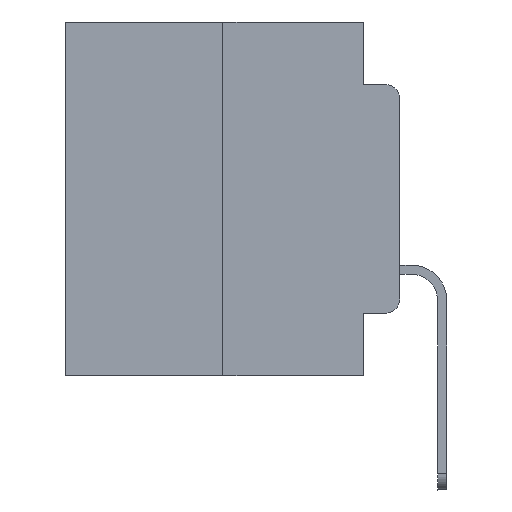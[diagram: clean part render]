
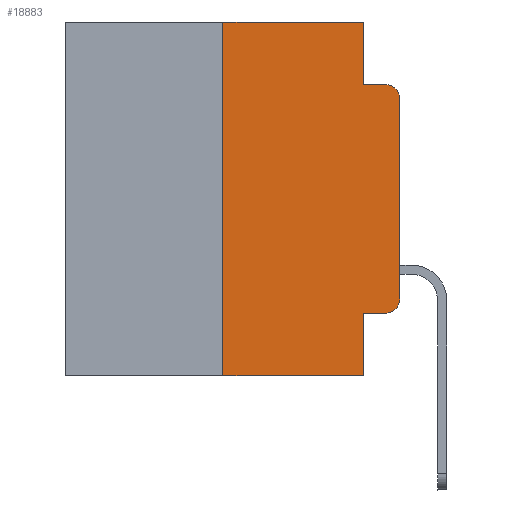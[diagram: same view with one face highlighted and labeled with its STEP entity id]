
A CAD part, left-side view. The second image highlights one B-rep face of the part: STEP entity #18883.
In plain terms, the highlighted planar face has unit normal (-1, 0, 0).
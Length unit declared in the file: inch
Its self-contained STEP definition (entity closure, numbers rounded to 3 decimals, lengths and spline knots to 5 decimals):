
#120 = ORIENTED_EDGE ( 'NONE', *, *, #20739, .F. ) ;
#444 = CARTESIAN_POINT ( 'NONE',  ( 0., 0.051, -0.5 ) ) ;
#709 = CARTESIAN_POINT ( 'NONE',  ( 0., 0.051, 0. ) ) ;
#1306 = LINE ( 'NONE', #9138, #14247 ) ;
#1525 = CARTESIAN_POINT ( 'NONE',  ( 0., 0., 0. ) ) ;
#1814 = CARTESIAN_POINT ( 'NONE',  ( 0., 0.25, 0. ) ) ;
#2393 = CARTESIAN_POINT ( 'NONE',  ( 0., 0.25, 0. ) ) ;
#2471 = LINE ( 'NONE', #709, #6243 ) ;
#2552 = CARTESIAN_POINT ( 'NONE',  ( 0., 0.473, 0. ) ) ;
#2804 = DIRECTION ( 'NONE',  ( 0., -1., 0. ) ) ;
#3104 = DIRECTION ( 'NONE',  ( -1., 0., 0. ) ) ;
#3635 = VECTOR ( 'NONE', #7529, 39.37008 ) ;
#3682 = VERTEX_POINT ( 'NONE', #25194 ) ;
#3683 = CIRCLE ( 'NONE', #25089, 0.02 ) ;
#4074 = EDGE_CURVE ( 'NONE', #9581, #21880, #10530, .T. ) ;
#4593 = AXIS2_PLACEMENT_3D ( 'NONE', #2552, #11045, #15161 ) ;
#5285 = CARTESIAN_POINT ( 'NONE',  ( 0., 0.051, 0. ) ) ;
#5499 = DIRECTION ( 'NONE',  ( 0., 0., 1. ) ) ;
#5785 = EDGE_LOOP ( 'NONE', ( #20632, #6701, #24751, #120, #11892, #18274, #25851, #20589, #6083, #16116 ) ) ;
#5890 = LINE ( 'NONE', #24358, #3635 ) ;
#6083 = ORIENTED_EDGE ( 'NONE', *, *, #4074, .T. ) ;
#6086 = VERTEX_POINT ( 'NONE', #444 ) ;
#6243 = VECTOR ( 'NONE', #25735, 39.37008 ) ;
#6701 = ORIENTED_EDGE ( 'NONE', *, *, #10238, .T. ) ;
#6797 = PLANE ( 'NONE',  #4593 ) ;
#7368 = LINE ( 'NONE', #17784, #16890 ) ;
#7529 = DIRECTION ( 'NONE',  ( 0., -1., 0. ) ) ;
#7711 = EDGE_CURVE ( 'NONE', #21880, #23110, #9277, .T. ) ;
#7956 = VERTEX_POINT ( 'NONE', #2393 ) ;
#7983 = VECTOR ( 'NONE', #11688, 39.37008 ) ;
#9138 = CARTESIAN_POINT ( 'NONE',  ( 0., 0.473, 0. ) ) ;
#9277 = CIRCLE ( 'NONE', #18892, 0.02 ) ;
#9518 = VECTOR ( 'NONE', #5499, 39.37008 ) ;
#9581 = VERTEX_POINT ( 'NONE', #14567 ) ;
#10238 = EDGE_CURVE ( 'NONE', #3682, #25160, #3683, .T. ) ;
#10530 = LINE ( 'NONE', #12851, #24457 ) ;
#11045 = DIRECTION ( 'NONE',  ( 1., 0., 0. ) ) ;
#11297 = EDGE_CURVE ( 'NONE', #25356, #6086, #7368, .T. ) ;
#11463 = DIRECTION ( 'NONE',  ( 0., 0., -1. ) ) ;
#11688 = DIRECTION ( 'NONE',  ( 0., 0., 1. ) ) ;
#11733 = EDGE_CURVE ( 'NONE', #7956, #15572, #1306, .T. ) ;
#11892 = ORIENTED_EDGE ( 'NONE', *, *, #11733, .F. ) ;
#12020 = DIRECTION ( 'NONE',  ( 0., 0., -1. ) ) ;
#12770 = CARTESIAN_POINT ( 'NONE',  ( 0., 0.051, -0.0885 ) ) ;
#12851 = CARTESIAN_POINT ( 'NONE',  ( 0., 0.051, -0.4115 ) ) ;
#13241 = CARTESIAN_POINT ( 'NONE',  ( 0., 0.02, -0.0885 ) ) ;
#13646 = DIRECTION ( 'NONE',  ( 0., 0., -1. ) ) ;
#13929 = CARTESIAN_POINT ( 'NONE',  ( 0., 0.02, -0.3915 ) ) ;
#14247 = VECTOR ( 'NONE', #2804, 39.37008 ) ;
#14567 = CARTESIAN_POINT ( 'NONE',  ( 0., 0.051, -0.4115 ) ) ;
#15161 = DIRECTION ( 'NONE',  ( 0., 0., -1. ) ) ;
#15572 = VERTEX_POINT ( 'NONE', #16154 ) ;
#15715 = DIRECTION ( 'NONE',  ( 0., -1., 0. ) ) ;
#16116 = ORIENTED_EDGE ( 'NONE', *, *, #7711, .T. ) ;
#16154 = CARTESIAN_POINT ( 'NONE',  ( 0., 0.051, 0. ) ) ;
#16483 = EDGE_CURVE ( 'NONE', #25356, #7956, #24387, .T. ) ;
#16890 = VECTOR ( 'NONE', #15715, 39.37008 ) ;
#16984 = EDGE_CURVE ( 'NONE', #17987, #25160, #5890, .T. ) ;
#17784 = CARTESIAN_POINT ( 'NONE',  ( 0., 0.473, -0.5 ) ) ;
#17890 = LINE ( 'NONE', #5285, #25546 ) ;
#17987 = VERTEX_POINT ( 'NONE', #12770 ) ;
#18042 = CARTESIAN_POINT ( 'NONE',  ( 0., 0.02, -0.1085 ) ) ;
#18274 = ORIENTED_EDGE ( 'NONE', *, *, #16483, .F. ) ;
#18883 = ADVANCED_FACE ( 'NONE', ( #23219 ), #6797, .F. ) ;
#18892 = AXIS2_PLACEMENT_3D ( 'NONE', #13929, #3104, #11463 ) ;
#19037 = EDGE_CURVE ( 'NONE', #9581, #6086, #17890, .T. ) ;
#20270 = LINE ( 'NONE', #1525, #9518 ) ;
#20589 = ORIENTED_EDGE ( 'NONE', *, *, #19037, .F. ) ;
#20632 = ORIENTED_EDGE ( 'NONE', *, *, #26118, .T. ) ;
#20739 = EDGE_CURVE ( 'NONE', #15572, #17987, #2471, .T. ) ;
#20972 = CARTESIAN_POINT ( 'NONE',  ( 0., 0., -0.3915 ) ) ;
#21013 = CARTESIAN_POINT ( 'NONE',  ( 0., 0.25, -0.5 ) ) ;
#21880 = VERTEX_POINT ( 'NONE', #23279 ) ;
#21991 = DIRECTION ( 'NONE',  ( -1., 0., 0. ) ) ;
#23110 = VERTEX_POINT ( 'NONE', #20972 ) ;
#23219 = FACE_OUTER_BOUND ( 'NONE', #5785, .T. ) ;
#23279 = CARTESIAN_POINT ( 'NONE',  ( 0., 0.02, -0.4115 ) ) ;
#24358 = CARTESIAN_POINT ( 'NONE',  ( 0., 0.051, -0.0885 ) ) ;
#24387 = LINE ( 'NONE', #1814, #7983 ) ;
#24457 = VECTOR ( 'NONE', #25157, 39.37008 ) ;
#24751 = ORIENTED_EDGE ( 'NONE', *, *, #16984, .F. ) ;
#25089 = AXIS2_PLACEMENT_3D ( 'NONE', #18042, #21991, #12020 ) ;
#25157 = DIRECTION ( 'NONE',  ( 0., -1., 0. ) ) ;
#25160 = VERTEX_POINT ( 'NONE', #13241 ) ;
#25194 = CARTESIAN_POINT ( 'NONE',  ( 0., 0., -0.1085 ) ) ;
#25356 = VERTEX_POINT ( 'NONE', #21013 ) ;
#25546 = VECTOR ( 'NONE', #13646, 39.37008 ) ;
#25735 = DIRECTION ( 'NONE',  ( 0., 0., -1. ) ) ;
#25851 = ORIENTED_EDGE ( 'NONE', *, *, #11297, .T. ) ;
#26118 = EDGE_CURVE ( 'NONE', #23110, #3682, #20270, .T. ) ;
